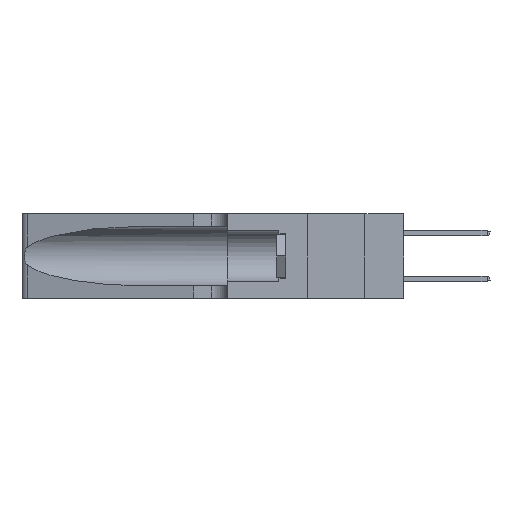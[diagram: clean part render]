
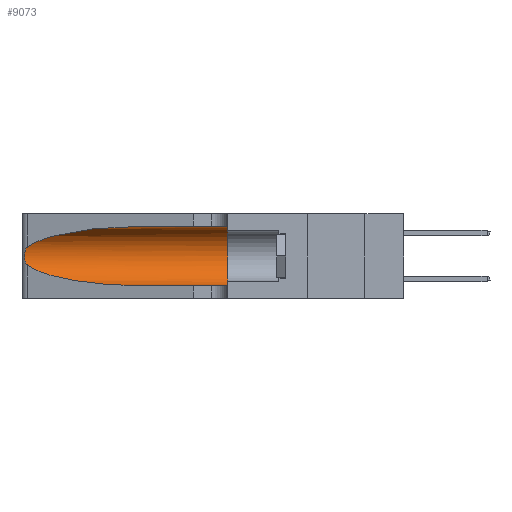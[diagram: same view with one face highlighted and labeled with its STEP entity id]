
A CAD part, left-side view. The second image highlights one B-rep face of the part: STEP entity #9073.
In plain terms, the highlighted cylindrical face has radius 3.308 mm (diameter 6.617 mm), a partial arc.
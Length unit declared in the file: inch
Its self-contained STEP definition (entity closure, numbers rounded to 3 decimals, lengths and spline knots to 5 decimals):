
#331 = CARTESIAN_POINT ( 'NONE',  ( 0.1305, 0.72297, 0.05475 ) ) ;
#455 = ORIENTED_EDGE ( 'NONE', *, *, #28403, .T. ) ;
#461 = CARTESIAN_POINT ( 'NONE',  ( 0.25487, 1.22718, 0.22369 ) ) ;
#508 = AXIS2_PLACEMENT_3D ( 'NONE', #24206, #9463, #30155 ) ;
#586 = CARTESIAN_POINT ( 'NONE',  ( 0.26075, 1.23896, 0.19203 ) ) ;
#2125 = CARTESIAN_POINT ( 'NONE',  ( 0.1305, 0.72297, 0.31525 ) ) ;
#2481 = CARTESIAN_POINT ( 'NONE',  ( 0.1305, 0.35, 0.05475 ) ) ;
#2758 = VERTEX_POINT ( 'NONE', #10613 ) ;
#2883 = VERTEX_POINT ( 'NONE', #2125 ) ;
#3208 = CARTESIAN_POINT ( 'NONE',  ( 0.2373, 1.15595, 0.28018 ) ) ;
#3322 =( BOUNDED_CURVE ( )  B_SPLINE_CURVE ( 3, ( #23213, #20263, #26178, #8428 ),
 .UNSPECIFIED., .F., .F. ) 
 B_SPLINE_CURVE_WITH_KNOTS ( ( 4, 4 ),
 ( 3.44316, 4.71239 ),
 .UNSPECIFIED. ) 
 CURVE ( )  GEOMETRIC_REPRESENTATION_ITEM ( )  RATIONAL_B_SPLINE_CURVE ( ( 1., 0.87, 0.87, 1. ) ) 
 REPRESENTATION_ITEM ( '' )  );
#3611 = DIRECTION ( 'NONE',  ( 0., 1., 0. ) ) ;
#3637 = CARTESIAN_POINT ( 'NONE',  ( 0.26017, 1.23833, 0.17102 ) ) ;
#4584 = CARTESIAN_POINT ( 'NONE',  ( 0.1305, 1.61858, 0.05475 ) ) ;
#4705 = VERTEX_POINT ( 'NONE', #2481 ) ;
#4925 = FACE_OUTER_BOUND ( 'NONE', #7811, .T. ) ;
#5410 = CARTESIAN_POINT ( 'NONE',  ( 0.25487, 1.22718, 0.14631 ) ) ;
#5633 = EDGE_CURVE ( 'NONE', #2758, #4705, #23332, .T. ) ;
#6031 = AXIS2_PLACEMENT_3D ( 'NONE', #21525, #3611, #24476 ) ;
#6692 = CARTESIAN_POINT ( 'NONE',  ( 0.25789, 1.23486, 0.15765 ) ) ;
#7811 = EDGE_LOOP ( 'NONE', ( #455, #9674, #9955, #20509, #12291, #9467 ) ) ;
#8428 = CARTESIAN_POINT ( 'NONE',  ( 0.1305, 0.72297, 0.05475 ) ) ;
#8662 = EDGE_CURVE ( 'NONE', #18685, #4705, #19926, .T. ) ;
#9073 = ADVANCED_FACE ( 'NONE', ( #4925 ), #18973, .F. ) ;
#9463 = DIRECTION ( 'NONE',  ( 0., -1., 0. ) ) ;
#9467 = ORIENTED_EDGE ( 'NONE', *, *, #17160, .F. ) ;
#9674 = ORIENTED_EDGE ( 'NONE', *, *, #28172, .T. ) ;
#9746 = CARTESIAN_POINT ( 'NONE',  ( 0.25555, 1.22993, 0.14849 ) ) ;
#9955 = ORIENTED_EDGE ( 'NONE', *, *, #21247, .T. ) ;
#10613 = CARTESIAN_POINT ( 'NONE',  ( 0.1305, 0.35, 0.31525 ) ) ;
#11550 = CARTESIAN_POINT ( 'NONE',  ( 0.1305, 1.61858, 0.31525 ) ) ;
#12035 = VECTOR ( 'NONE', #37279, 39.37008 ) ;
#12291 = ORIENTED_EDGE ( 'NONE', *, *, #5633, .F. ) ;
#13906 =( BOUNDED_CURVE ( )  B_SPLINE_CURVE ( 3, ( #23934, #18174, #3208, #24063 ),
 .UNSPECIFIED., .F., .F. ) 
 B_SPLINE_CURVE_WITH_KNOTS ( ( 4, 4 ),
 ( 1.5708, 2.84003 ),
 .UNSPECIFIED. ) 
 CURVE ( )  GEOMETRIC_REPRESENTATION_ITEM ( )  RATIONAL_B_SPLINE_CURVE ( ( 1., 0.87, 0.87, 1. ) ) 
 REPRESENTATION_ITEM ( '' )  );
#15577 = CARTESIAN_POINT ( 'NONE',  ( 0.25787, 1.23484, 0.2124 ) ) ;
#17160 = EDGE_CURVE ( 'NONE', #2883, #2758, #35030, .T. ) ;
#18174 = CARTESIAN_POINT ( 'NONE',  ( 0.18966, 0.96281, 0.31525 ) ) ;
#18592 = CARTESIAN_POINT ( 'NONE',  ( 0.26018, 1.23835, 0.19895 ) ) ;
#18685 = VERTEX_POINT ( 'NONE', #331 ) ;
#18973 = CYLINDRICAL_SURFACE ( 'NONE', #508, 0.13025 ) ;
#19926 = LINE ( 'NONE', #4584, #12035 ) ;
#20263 = CARTESIAN_POINT ( 'NONE',  ( 0.2373, 1.15595, 0.08982 ) ) ;
#20509 = ORIENTED_EDGE ( 'NONE', *, *, #8662, .T. ) ;
#21247 = EDGE_CURVE ( 'NONE', #36859, #18685, #3322, .T. ) ;
#21525 = CARTESIAN_POINT ( 'NONE',  ( 0.1305, 0.35, 0.185 ) ) ;
#21554 = CARTESIAN_POINT ( 'NONE',  ( 0.26075, 1.23896, 0.178 ) ) ;
#23213 = CARTESIAN_POINT ( 'NONE',  ( 0.25487, 1.22718, 0.14631 ) ) ;
#23332 = CIRCLE ( 'NONE', #6031, 0.13025 ) ;
#23934 = CARTESIAN_POINT ( 'NONE',  ( 0.1305, 0.72297, 0.31525 ) ) ;
#24063 = CARTESIAN_POINT ( 'NONE',  ( 0.25487, 1.22718, 0.22369 ) ) ;
#24206 = CARTESIAN_POINT ( 'NONE',  ( 0.1305, 1.61858, 0.185 ) ) ;
#24361 = CARTESIAN_POINT ( 'NONE',  ( 0.25555, 1.22994, 0.2215 ) ) ;
#24476 = DIRECTION ( 'NONE',  ( 0., 0., 1. ) ) ;
#24496 = CARTESIAN_POINT ( 'NONE',  ( 0.25856, 1.23593, 0.16098 ) ) ;
#26178 = CARTESIAN_POINT ( 'NONE',  ( 0.18966, 0.96281, 0.05475 ) ) ;
#26200 = VECTOR ( 'NONE', #35230, 39.37008 ) ;
#27462 = CARTESIAN_POINT ( 'NONE',  ( 0.25639, 1.23186, 0.15144 ) ) ;
#28172 = EDGE_CURVE ( 'NONE', #33593, #36859, #35660, .T. ) ;
#28403 = EDGE_CURVE ( 'NONE', #2883, #33593, #13906, .T. ) ;
#30155 = DIRECTION ( 'NONE',  ( 0., 0., -1. ) ) ;
#30440 = CARTESIAN_POINT ( 'NONE',  ( 0.25487, 1.22718, 0.14631 ) ) ;
#33330 = CARTESIAN_POINT ( 'NONE',  ( 0.25639, 1.23184, 0.21858 ) ) ;
#33593 = VERTEX_POINT ( 'NONE', #37175 ) ;
#35030 = LINE ( 'NONE', #11550, #26200 ) ;
#35230 = DIRECTION ( 'NONE',  ( 0., -1., 0. ) ) ;
#35660 = B_SPLINE_CURVE_WITH_KNOTS ( 'NONE', 3,
 ( #461, #24361, #33330, #15577, #36266, #18592, #586, #21554, #3637, #24496, #6692, #27462, #9746, #30440 ),
 .UNSPECIFIED., .F., .F.,
 ( 4, 2, 2, 2, 2, 2, 4 ),
 ( 0., 0.00027, 0.00053, 0.00107, 0.0016, 0.00187, 0.00214 ),
 .UNSPECIFIED. ) ;
#36266 = CARTESIAN_POINT ( 'NONE',  ( 0.25854, 1.2359, 0.20912 ) ) ;
#36859 = VERTEX_POINT ( 'NONE', #5410 ) ;
#37175 = CARTESIAN_POINT ( 'NONE',  ( 0.25487, 1.22718, 0.22369 ) ) ;
#37279 = DIRECTION ( 'NONE',  ( 0., -1., 0. ) ) ;
